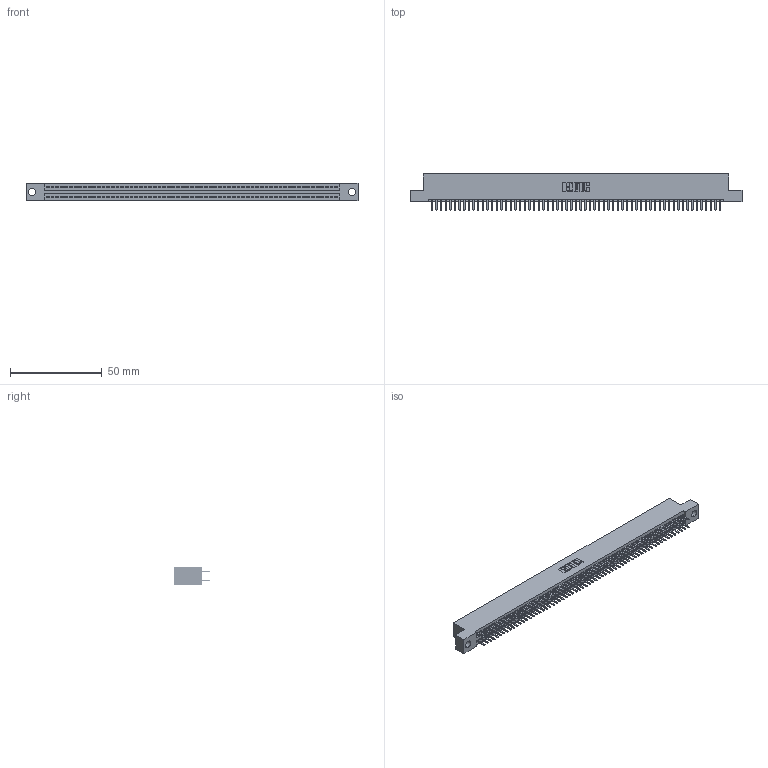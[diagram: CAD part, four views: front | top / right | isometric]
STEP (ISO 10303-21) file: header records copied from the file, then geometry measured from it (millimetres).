
FILE_DESCRIPTION (( 'STEP AP203' ), '1' );
FILE_NAME ('395-126-520-204.STEP', '2021-06-17T22:35:02', ( '' ), ( '' ), 'SwSTEP 2.0', 'SolidWorks 2020', '' );
FILE_SCHEMA (( 'CONFIG_CONTROL_DESIGN' ));
Length unit declared in the file: inch
Products named in the file (3): 395-126-520-204; 345-292-001_345-293-120; 345 Part_Flush Mounting Lugs - 0.156 Dia-TI
Assembly tree (127 placements, depth 2):
  395-126-520-204
    345 Part_Flush Mounting Lugs - 0.156 Dia-TI
    345-292-001_345-293-120  x126
Bounding box: 181.23 x 19.68 x 9.4 mm (x, y, z)
Volume: 17638.4 mm3; surface area: 26213 mm2
Topology: 127 solids, 127 shells, 6944 faces, 20159 edges, 13102 vertices
Faces by surface type: plane 4504, cylinder 2440
Entity records: 47137 total; most frequent: CARTESIAN_POINT 7898, ORIENTED_EDGE 7818, DIRECTION 6925, EDGE_CURVE 3909, LINE 3521, VECTOR 3521, VERTEX_POINT 2602, AXIS2_PLACEMENT_3D 1702
